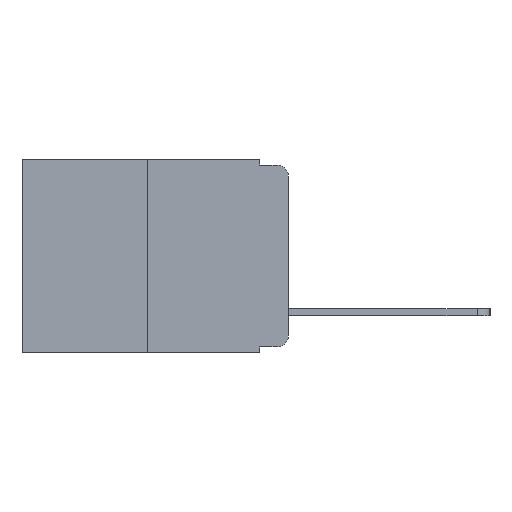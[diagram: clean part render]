
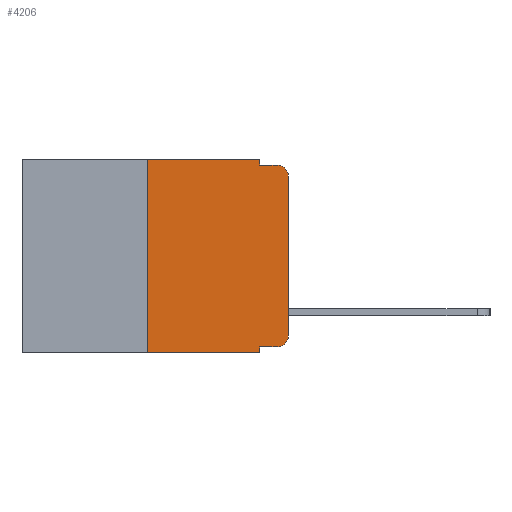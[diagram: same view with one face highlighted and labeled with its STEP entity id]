
A CAD part, left-side view. The second image highlights one B-rep face of the part: STEP entity #4206.
In plain terms, the highlighted planar face has unit normal (-1, 0, 0).
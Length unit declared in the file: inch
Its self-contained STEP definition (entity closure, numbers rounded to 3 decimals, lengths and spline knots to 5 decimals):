
#400 = CARTESIAN_POINT ( 'NONE',  ( 0., 0.02, -0.333 ) ) ;
#401 = DIRECTION ( 'NONE',  ( -1., 0., 0. ) ) ;
#552 = LINE ( 'NONE', #13893, #8052 ) ;
#637 = ORIENTED_EDGE ( 'NONE', *, *, #2938, .T. ) ;
#901 = EDGE_CURVE ( 'NONE', #12854, #1031, #552, .T. ) ;
#1031 = VERTEX_POINT ( 'NONE', #15945 ) ;
#1106 = VERTEX_POINT ( 'NONE', #2065 ) ;
#1174 = AXIS2_PLACEMENT_3D ( 'NONE', #12368, #4008, #13676 ) ;
#1370 = VERTEX_POINT ( 'NONE', #5983 ) ;
#1949 = LINE ( 'NONE', #2787, #9299 ) ;
#2065 = CARTESIAN_POINT ( 'NONE',  ( 0., 0.25, -0.343 ) ) ;
#2787 = CARTESIAN_POINT ( 'NONE',  ( 0., 0., 0. ) ) ;
#2938 = EDGE_CURVE ( 'NONE', #3462, #1031, #5405, .T. ) ;
#3462 = VERTEX_POINT ( 'NONE', #9617 ) ;
#3711 = CARTESIAN_POINT ( 'NONE',  ( 0., 0.051, 0. ) ) ;
#3818 = DIRECTION ( 'NONE',  ( 0., 0., -1. ) ) ;
#4008 = DIRECTION ( 'NONE',  ( -1., 0., 0. ) ) ;
#4052 = AXIS2_PLACEMENT_3D ( 'NONE', #9242, #401, #10581 ) ;
#4156 = CARTESIAN_POINT ( 'NONE',  ( 0., 0.051, -0.333 ) ) ;
#4206 = ADVANCED_FACE ( 'NONE', ( #5289 ), #7883, .F. ) ;
#4261 = DIRECTION ( 'NONE',  ( 0., 0., 1. ) ) ;
#4870 = CARTESIAN_POINT ( 'NONE',  ( 0., 0.473, 0. ) ) ;
#4905 = EDGE_CURVE ( 'NONE', #12719, #3462, #1949, .T. ) ;
#5289 = FACE_OUTER_BOUND ( 'NONE', #12827, .T. ) ;
#5405 = CIRCLE ( 'NONE', #4052, 0.02 ) ;
#5464 = CARTESIAN_POINT ( 'NONE',  ( 0., 0.051, 0. ) ) ;
#5551 = ORIENTED_EDGE ( 'NONE', *, *, #17839, .F. ) ;
#5983 = CARTESIAN_POINT ( 'NONE',  ( 0., 0.051, 0. ) ) ;
#6020 = ORIENTED_EDGE ( 'NONE', *, *, #11060, .F. ) ;
#6042 = CARTESIAN_POINT ( 'NONE',  ( 0., 0., -0.313 ) ) ;
#6236 = CARTESIAN_POINT ( 'NONE',  ( 0., 0.473, 0. ) ) ;
#6269 = VECTOR ( 'NONE', #11407, 39.37008 ) ;
#6302 = CARTESIAN_POINT ( 'NONE',  ( 0., 0.051, -0.01 ) ) ;
#6996 = DIRECTION ( 'NONE',  ( 0., 0., -1. ) ) ;
#7060 = VECTOR ( 'NONE', #12060, 39.37008 ) ;
#7080 = VERTEX_POINT ( 'NONE', #8131 ) ;
#7245 = VERTEX_POINT ( 'NONE', #4156 ) ;
#7440 = ORIENTED_EDGE ( 'NONE', *, *, #14461, .F. ) ;
#7702 = LINE ( 'NONE', #6236, #14349 ) ;
#7731 = DIRECTION ( 'NONE',  ( 0., -1., 0. ) ) ;
#7883 = PLANE ( 'NONE',  #14488 ) ;
#8052 = VECTOR ( 'NONE', #9588, 39.37008 ) ;
#8131 = CARTESIAN_POINT ( 'NONE',  ( 0., 0.25, 0. ) ) ;
#8657 = VECTOR ( 'NONE', #3818, 39.37008 ) ;
#8869 = CARTESIAN_POINT ( 'NONE',  ( 0., 0.25, 0. ) ) ;
#8965 = ORIENTED_EDGE ( 'NONE', *, *, #901, .F. ) ;
#9233 = DIRECTION ( 'NONE',  ( 0., 0., -1. ) ) ;
#9242 = CARTESIAN_POINT ( 'NONE',  ( 0., 0.02, -0.03 ) ) ;
#9299 = VECTOR ( 'NONE', #4261, 39.37008 ) ;
#9588 = DIRECTION ( 'NONE',  ( 0., -1., 0. ) ) ;
#9617 = CARTESIAN_POINT ( 'NONE',  ( 0., 0., -0.03 ) ) ;
#9805 = ORIENTED_EDGE ( 'NONE', *, *, #16143, .F. ) ;
#10084 = CARTESIAN_POINT ( 'NONE',  ( 0., 0.051, -0.333 ) ) ;
#10209 = DIRECTION ( 'NONE',  ( 0., 0., 1. ) ) ;
#10213 = ORIENTED_EDGE ( 'NONE', *, *, #15521, .T. ) ;
#10581 = DIRECTION ( 'NONE',  ( 0., 0., -1. ) ) ;
#10684 = LINE ( 'NONE', #17162, #7060 ) ;
#10922 = EDGE_CURVE ( 'NONE', #12899, #12719, #15939, .T. ) ;
#11060 = EDGE_CURVE ( 'NONE', #7080, #1370, #7702, .T. ) ;
#11241 = ORIENTED_EDGE ( 'NONE', *, *, #4905, .T. ) ;
#11407 = DIRECTION ( 'NONE',  ( 0., -1., 0. ) ) ;
#11441 = ORIENTED_EDGE ( 'NONE', *, *, #10922, .T. ) ;
#11808 = EDGE_CURVE ( 'NONE', #7245, #12899, #13496, .T. ) ;
#12060 = DIRECTION ( 'NONE',  ( 0., -1., 0. ) ) ;
#12368 = CARTESIAN_POINT ( 'NONE',  ( 0., 0.02, -0.313 ) ) ;
#12719 = VERTEX_POINT ( 'NONE', #6042 ) ;
#12827 = EDGE_LOOP ( 'NONE', ( #11241, #637, #8965, #5551, #6020, #9805, #10213, #7440, #14539, #11441 ) ) ;
#12854 = VERTEX_POINT ( 'NONE', #6302 ) ;
#12899 = VERTEX_POINT ( 'NONE', #400 ) ;
#13496 = LINE ( 'NONE', #10084, #6269 ) ;
#13676 = DIRECTION ( 'NONE',  ( 0., 0., -1. ) ) ;
#13780 = LINE ( 'NONE', #3711, #8657 ) ;
#13893 = CARTESIAN_POINT ( 'NONE',  ( 0., 0.051, -0.01 ) ) ;
#14349 = VECTOR ( 'NONE', #7731, 39.37008 ) ;
#14461 = EDGE_CURVE ( 'NONE', #7245, #16592, #13780, .T. ) ;
#14488 = AXIS2_PLACEMENT_3D ( 'NONE', #4870, #16999, #9233 ) ;
#14539 = ORIENTED_EDGE ( 'NONE', *, *, #11808, .T. ) ;
#14580 = VECTOR ( 'NONE', #10209, 39.37008 ) ;
#14985 = LINE ( 'NONE', #8869, #14580 ) ;
#15150 = LINE ( 'NONE', #5464, #17702 ) ;
#15521 = EDGE_CURVE ( 'NONE', #1106, #16592, #10684, .T. ) ;
#15939 = CIRCLE ( 'NONE', #1174, 0.02 ) ;
#15945 = CARTESIAN_POINT ( 'NONE',  ( 0., 0.02, -0.01 ) ) ;
#16143 = EDGE_CURVE ( 'NONE', #1106, #7080, #14985, .T. ) ;
#16592 = VERTEX_POINT ( 'NONE', #17263 ) ;
#16999 = DIRECTION ( 'NONE',  ( 1., 0., 0. ) ) ;
#17162 = CARTESIAN_POINT ( 'NONE',  ( 0., 0.473, -0.343 ) ) ;
#17263 = CARTESIAN_POINT ( 'NONE',  ( 0., 0.051, -0.343 ) ) ;
#17702 = VECTOR ( 'NONE', #6996, 39.37008 ) ;
#17839 = EDGE_CURVE ( 'NONE', #1370, #12854, #15150, .T. ) ;
